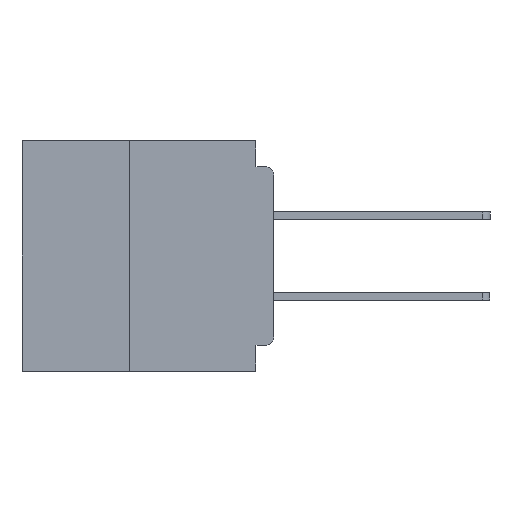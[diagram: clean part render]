
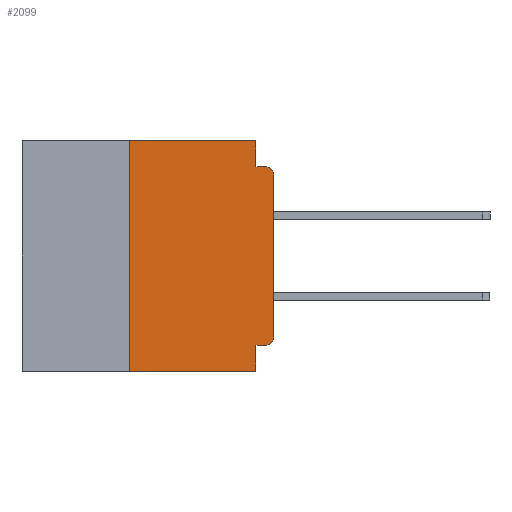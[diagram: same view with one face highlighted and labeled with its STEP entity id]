
A CAD part, left-side view. The second image highlights one B-rep face of the part: STEP entity #2099.
In plain terms, the highlighted planar face has unit normal (-1, 0, 0).
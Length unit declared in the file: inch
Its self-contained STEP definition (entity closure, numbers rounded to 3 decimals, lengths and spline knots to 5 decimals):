
#659 = EDGE_CURVE ( 'NONE', #30950, #1596, #39589, .T. ) ;
#1251 = ORIENTED_EDGE ( 'NONE', *, *, #15584, .T. ) ;
#1256 = VERTEX_POINT ( 'NONE', #15287 ) ;
#1363 = LINE ( 'NONE', #36890, #38707 ) ;
#1596 = VERTEX_POINT ( 'NONE', #37320 ) ;
#1969 = VERTEX_POINT ( 'NONE', #4202 ) ;
#2099 = ADVANCED_FACE ( 'NONE', ( #6602 ), #36716, .F. ) ;
#4202 = CARTESIAN_POINT ( 'NONE',  ( 0., 0.031, 0. ) ) ;
#4413 = CARTESIAN_POINT ( 'NONE',  ( 0., 0.031, -0.045 ) ) ;
#6222 = EDGE_LOOP ( 'NONE', ( #7795, #43721, #20465, #14857, #18823, #31609, #21826, #18149, #43289, #1251 ) ) ;
#6444 = CARTESIAN_POINT ( 'NONE',  ( 0., 0.031, -0.4 ) ) ;
#6602 = FACE_OUTER_BOUND ( 'NONE', #6222, .T. ) ;
#6630 = CARTESIAN_POINT ( 'NONE',  ( 0., 0.25, 0. ) ) ;
#6732 = EDGE_CURVE ( 'NONE', #1256, #13668, #17778, .T. ) ;
#7795 = ORIENTED_EDGE ( 'NONE', *, *, #659, .T. ) ;
#9481 = CARTESIAN_POINT ( 'NONE',  ( 0., 0.25, -0.4 ) ) ;
#9932 = VECTOR ( 'NONE', #36371, 39.37008 ) ;
#10723 = EDGE_CURVE ( 'NONE', #13900, #13668, #16353, .T. ) ;
#10841 = DIRECTION ( 'NONE',  ( -1., 0., 0. ) ) ;
#10980 = CARTESIAN_POINT ( 'NONE',  ( 0., 0., -0.34 ) ) ;
#10989 = DIRECTION ( 'NONE',  ( 0., -1., 0. ) ) ;
#12299 = EDGE_CURVE ( 'NONE', #1969, #16590, #21721, .T. ) ;
#12375 = VECTOR ( 'NONE', #41440, 39.37008 ) ;
#13668 = VERTEX_POINT ( 'NONE', #6444 ) ;
#13795 = EDGE_CURVE ( 'NONE', #16590, #35760, #45280, .T. ) ;
#13900 = VERTEX_POINT ( 'NONE', #15135 ) ;
#14857 = ORIENTED_EDGE ( 'NONE', *, *, #12299, .F. ) ;
#15135 = CARTESIAN_POINT ( 'NONE',  ( 0., 0.031, -0.355 ) ) ;
#15287 = CARTESIAN_POINT ( 'NONE',  ( 0., 0.25, -0.4 ) ) ;
#15584 = EDGE_CURVE ( 'NONE', #28585, #30950, #33686, .T. ) ;
#16332 = AXIS2_PLACEMENT_3D ( 'NONE', #31780, #10841, #35298 ) ;
#16353 = LINE ( 'NONE', #43281, #40916 ) ;
#16590 = VERTEX_POINT ( 'NONE', #4413 ) ;
#17778 = LINE ( 'NONE', #19604, #25971 ) ;
#18149 = ORIENTED_EDGE ( 'NONE', *, *, #10723, .F. ) ;
#18403 = VECTOR ( 'NONE', #26938, 39.37008 ) ;
#18442 = CARTESIAN_POINT ( 'NONE',  ( 0., 0.015, -0.06 ) ) ;
#18823 = ORIENTED_EDGE ( 'NONE', *, *, #24015, .F. ) ;
#19492 = LINE ( 'NONE', #9481, #18403 ) ;
#19604 = CARTESIAN_POINT ( 'NONE',  ( 0., 0.437, -0.4 ) ) ;
#20275 = CARTESIAN_POINT ( 'NONE',  ( 0., 0.031, 0. ) ) ;
#20465 = ORIENTED_EDGE ( 'NONE', *, *, #13795, .F. ) ;
#21051 = VECTOR ( 'NONE', #42448, 39.37008 ) ;
#21412 = CARTESIAN_POINT ( 'NONE',  ( 0., 0., -0.045 ) ) ;
#21721 = LINE ( 'NONE', #20275, #12375 ) ;
#21826 = ORIENTED_EDGE ( 'NONE', *, *, #6732, .T. ) ;
#21962 = DIRECTION ( 'NONE',  ( 0., 0., -1. ) ) ;
#22202 = AXIS2_PLACEMENT_3D ( 'NONE', #18442, #42815, #21962 ) ;
#22513 = CARTESIAN_POINT ( 'NONE',  ( 0., 0., -0.355 ) ) ;
#23858 = CARTESIAN_POINT ( 'NONE',  ( 0., 0.015, -0.045 ) ) ;
#24015 = EDGE_CURVE ( 'NONE', #26609, #1969, #1363, .T. ) ;
#25971 = VECTOR ( 'NONE', #40464, 39.37008 ) ;
#26529 = DIRECTION ( 'NONE',  ( 0., -1., 0. ) ) ;
#26609 = VERTEX_POINT ( 'NONE', #6630 ) ;
#26776 = VECTOR ( 'NONE', #10989, 39.37008 ) ;
#26938 = DIRECTION ( 'NONE',  ( 0., 0., 1. ) ) ;
#27461 = LINE ( 'NONE', #22513, #9932 ) ;
#28585 = VERTEX_POINT ( 'NONE', #29062 ) ;
#29062 = CARTESIAN_POINT ( 'NONE',  ( 0., 0.015, -0.355 ) ) ;
#29282 = DIRECTION ( 'NONE',  ( 0., 0., -1. ) ) ;
#29769 = EDGE_CURVE ( 'NONE', #1596, #35760, #37673, .T. ) ;
#29785 = CARTESIAN_POINT ( 'NONE',  ( 0., 0., 0. ) ) ;
#30950 = VERTEX_POINT ( 'NONE', #10980 ) ;
#31609 = ORIENTED_EDGE ( 'NONE', *, *, #35161, .F. ) ;
#31780 = CARTESIAN_POINT ( 'NONE',  ( 0., 0.015, -0.34 ) ) ;
#33507 = AXIS2_PLACEMENT_3D ( 'NONE', #36577, #36241, #29282 ) ;
#33686 = CIRCLE ( 'NONE', #16332, 0.015 ) ;
#35161 = EDGE_CURVE ( 'NONE', #1256, #26609, #19492, .T. ) ;
#35298 = DIRECTION ( 'NONE',  ( 0., 0., -1. ) ) ;
#35760 = VERTEX_POINT ( 'NONE', #23858 ) ;
#36241 = DIRECTION ( 'NONE',  ( 1., 0., 0. ) ) ;
#36371 = DIRECTION ( 'NONE',  ( 0., 1., 0. ) ) ;
#36577 = CARTESIAN_POINT ( 'NONE',  ( 0., 0.437, 0. ) ) ;
#36716 = PLANE ( 'NONE',  #33507 ) ;
#36890 = CARTESIAN_POINT ( 'NONE',  ( 0., 0.437, 0. ) ) ;
#37320 = CARTESIAN_POINT ( 'NONE',  ( 0., 0., -0.06 ) ) ;
#37673 = CIRCLE ( 'NONE', #22202, 0.015 ) ;
#38707 = VECTOR ( 'NONE', #26529, 39.37008 ) ;
#39589 = LINE ( 'NONE', #29785, #21051 ) ;
#40409 = EDGE_CURVE ( 'NONE', #28585, #13900, #27461, .T. ) ;
#40464 = DIRECTION ( 'NONE',  ( 0., -1., 0. ) ) ;
#40916 = VECTOR ( 'NONE', #43446, 39.37008 ) ;
#41440 = DIRECTION ( 'NONE',  ( 0., 0., -1. ) ) ;
#42448 = DIRECTION ( 'NONE',  ( 0., 0., 1. ) ) ;
#42815 = DIRECTION ( 'NONE',  ( -1., 0., 0. ) ) ;
#43281 = CARTESIAN_POINT ( 'NONE',  ( 0., 0.031, -0.4 ) ) ;
#43289 = ORIENTED_EDGE ( 'NONE', *, *, #40409, .F. ) ;
#43446 = DIRECTION ( 'NONE',  ( 0., 0., -1. ) ) ;
#43721 = ORIENTED_EDGE ( 'NONE', *, *, #29769, .T. ) ;
#45280 = LINE ( 'NONE', #21412, #26776 ) ;
